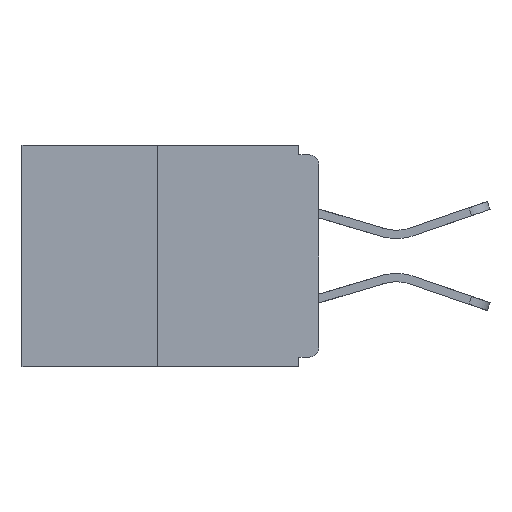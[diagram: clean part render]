
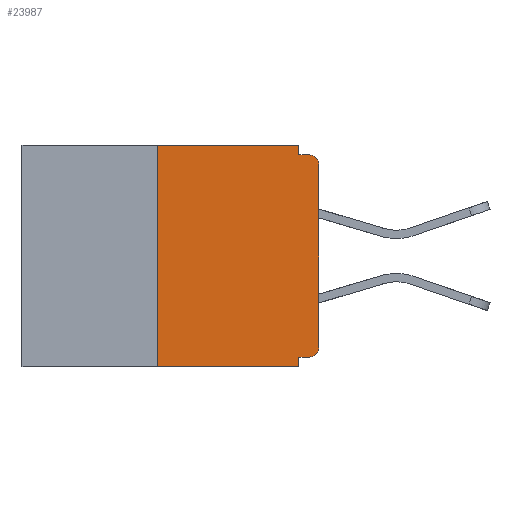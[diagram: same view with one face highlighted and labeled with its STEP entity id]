
A CAD part, left-side view. The second image highlights one B-rep face of the part: STEP entity #23987.
In plain terms, the highlighted planar face has unit normal (-1, 0, 0).
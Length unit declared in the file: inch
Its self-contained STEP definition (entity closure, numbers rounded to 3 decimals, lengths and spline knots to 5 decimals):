
#375 = VECTOR ( 'NONE', #1926, 39.37008 ) ;
#531 = ORIENTED_EDGE ( 'NONE', *, *, #1220, .T. ) ;
#916 = VERTEX_POINT ( 'NONE', #14608 ) ;
#1220 = EDGE_CURVE ( 'NONE', #22970, #12623, #9479, .T. ) ;
#1591 = DIRECTION ( 'NONE',  ( 0., 0., 1. ) ) ;
#1926 = DIRECTION ( 'NONE',  ( 0., -1., 0. ) ) ;
#1967 = VERTEX_POINT ( 'NONE', #14921 ) ;
#1988 = CARTESIAN_POINT ( 'NONE',  ( 0., 0., -0.328 ) ) ;
#2001 = DIRECTION ( 'NONE',  ( 0., 0., -1. ) ) ;
#2626 = CARTESIAN_POINT ( 'NONE',  ( 0., 0.031, 0. ) ) ;
#2994 = LINE ( 'NONE', #15260, #3600 ) ;
#3102 = EDGE_CURVE ( 'NONE', #916, #5421, #24294, .T. ) ;
#3600 = VECTOR ( 'NONE', #17225, 39.37008 ) ;
#3745 = AXIS2_PLACEMENT_3D ( 'NONE', #24382, #6548, #20255 ) ;
#3940 = VECTOR ( 'NONE', #1591, 39.37008 ) ;
#4170 = ORIENTED_EDGE ( 'NONE', *, *, #9101, .F. ) ;
#4235 = AXIS2_PLACEMENT_3D ( 'NONE', #23540, #11787, #23711 ) ;
#5331 = CARTESIAN_POINT ( 'NONE',  ( 0., 0.25, -0.343 ) ) ;
#5421 = VERTEX_POINT ( 'NONE', #20456 ) ;
#6409 = ORIENTED_EDGE ( 'NONE', *, *, #9284, .F. ) ;
#6548 = DIRECTION ( 'NONE',  ( -1., 0., 0. ) ) ;
#7038 = ORIENTED_EDGE ( 'NONE', *, *, #18784, .T. ) ;
#7258 = CARTESIAN_POINT ( 'NONE',  ( 0., 0.25, 0. ) ) ;
#7569 = LINE ( 'NONE', #7258, #23398 ) ;
#7704 = VECTOR ( 'NONE', #15703, 39.37008 ) ;
#8446 = ORIENTED_EDGE ( 'NONE', *, *, #14601, .F. ) ;
#8618 = ORIENTED_EDGE ( 'NONE', *, *, #3102, .T. ) ;
#8944 = DIRECTION ( 'NONE',  ( 0., -1., 0. ) ) ;
#9026 = CARTESIAN_POINT ( 'NONE',  ( 0., 0., -0.03 ) ) ;
#9045 = ORIENTED_EDGE ( 'NONE', *, *, #24065, .F. ) ;
#9101 = EDGE_CURVE ( 'NONE', #22970, #1967, #7569, .T. ) ;
#9178 = VERTEX_POINT ( 'NONE', #9026 ) ;
#9284 = EDGE_CURVE ( 'NONE', #1967, #24782, #2994, .T. ) ;
#9479 = LINE ( 'NONE', #13577, #375 ) ;
#9676 = ORIENTED_EDGE ( 'NONE', *, *, #19214, .F. ) ;
#9761 = CARTESIAN_POINT ( 'NONE',  ( 0., 0.031, -0.343 ) ) ;
#9789 = EDGE_LOOP ( 'NONE', ( #6409, #4170, #531, #24244, #9045, #8618, #11588, #7038, #9676, #8446 ) ) ;
#10309 = VERTEX_POINT ( 'NONE', #20670 ) ;
#11588 = ORIENTED_EDGE ( 'NONE', *, *, #11938, .T. ) ;
#11787 = DIRECTION ( 'NONE',  ( 1., 0., 0. ) ) ;
#11938 = EDGE_CURVE ( 'NONE', #5421, #9178, #15830, .T. ) ;
#12375 = VERTEX_POINT ( 'NONE', #20661 ) ;
#12623 = VERTEX_POINT ( 'NONE', #17374 ) ;
#13040 = CARTESIAN_POINT ( 'NONE',  ( 0., 0.031, 0. ) ) ;
#13296 = PLANE ( 'NONE',  #4235 ) ;
#13577 = CARTESIAN_POINT ( 'NONE',  ( 0., 0.46, -0.343 ) ) ;
#14133 = VECTOR ( 'NONE', #2001, 39.37008 ) ;
#14213 = CARTESIAN_POINT ( 'NONE',  ( 0., 0., -0.015 ) ) ;
#14566 = AXIS2_PLACEMENT_3D ( 'NONE', #14893, #24750, #18759 ) ;
#14601 = EDGE_CURVE ( 'NONE', #24782, #10309, #24068, .T. ) ;
#14608 = CARTESIAN_POINT ( 'NONE',  ( 0., 0.015, -0.328 ) ) ;
#14893 = CARTESIAN_POINT ( 'NONE',  ( 0., 0.015, -0.03 ) ) ;
#14921 = CARTESIAN_POINT ( 'NONE',  ( 0., 0.25, 0. ) ) ;
#15260 = CARTESIAN_POINT ( 'NONE',  ( 0., 0.46, 0. ) ) ;
#15703 = DIRECTION ( 'NONE',  ( 0., 1., 0. ) ) ;
#15710 = VECTOR ( 'NONE', #8944, 39.37008 ) ;
#15830 = LINE ( 'NONE', #21287, #3940 ) ;
#15862 = VECTOR ( 'NONE', #16234, 39.37008 ) ;
#16234 = DIRECTION ( 'NONE',  ( 0., 0., -1. ) ) ;
#17225 = DIRECTION ( 'NONE',  ( 0., -1., 0. ) ) ;
#17374 = CARTESIAN_POINT ( 'NONE',  ( 0., 0.031, -0.343 ) ) ;
#18078 = FACE_OUTER_BOUND ( 'NONE', #9789, .T. ) ;
#18667 = LINE ( 'NONE', #1988, #7704 ) ;
#18759 = DIRECTION ( 'NONE',  ( 0., 0., -1. ) ) ;
#18784 = EDGE_CURVE ( 'NONE', #9178, #20479, #19375, .T. ) ;
#19214 = EDGE_CURVE ( 'NONE', #10309, #20479, #21522, .T. ) ;
#19375 = CIRCLE ( 'NONE', #14566, 0.015 ) ;
#19971 = EDGE_CURVE ( 'NONE', #12375, #12623, #24463, .T. ) ;
#20255 = DIRECTION ( 'NONE',  ( 0., 0., -1. ) ) ;
#20456 = CARTESIAN_POINT ( 'NONE',  ( 0., 0., -0.313 ) ) ;
#20479 = VERTEX_POINT ( 'NONE', #24979 ) ;
#20661 = CARTESIAN_POINT ( 'NONE',  ( 0., 0.031, -0.328 ) ) ;
#20670 = CARTESIAN_POINT ( 'NONE',  ( 0., 0.031, -0.015 ) ) ;
#21287 = CARTESIAN_POINT ( 'NONE',  ( 0., 0., 0. ) ) ;
#21522 = LINE ( 'NONE', #14213, #15710 ) ;
#22831 = DIRECTION ( 'NONE',  ( 0., 0., 1. ) ) ;
#22970 = VERTEX_POINT ( 'NONE', #5331 ) ;
#23398 = VECTOR ( 'NONE', #22831, 39.37008 ) ;
#23540 = CARTESIAN_POINT ( 'NONE',  ( 0., 0.46, 0. ) ) ;
#23711 = DIRECTION ( 'NONE',  ( 0., 0., -1. ) ) ;
#23987 = ADVANCED_FACE ( 'NONE', ( #18078 ), #13296, .F. ) ;
#24065 = EDGE_CURVE ( 'NONE', #916, #12375, #18667, .T. ) ;
#24068 = LINE ( 'NONE', #2626, #15862 ) ;
#24244 = ORIENTED_EDGE ( 'NONE', *, *, #19971, .F. ) ;
#24294 = CIRCLE ( 'NONE', #3745, 0.015 ) ;
#24382 = CARTESIAN_POINT ( 'NONE',  ( 0., 0.015, -0.313 ) ) ;
#24463 = LINE ( 'NONE', #9761, #14133 ) ;
#24750 = DIRECTION ( 'NONE',  ( -1., 0., 0. ) ) ;
#24782 = VERTEX_POINT ( 'NONE', #13040 ) ;
#24979 = CARTESIAN_POINT ( 'NONE',  ( 0., 0.015, -0.015 ) ) ;
